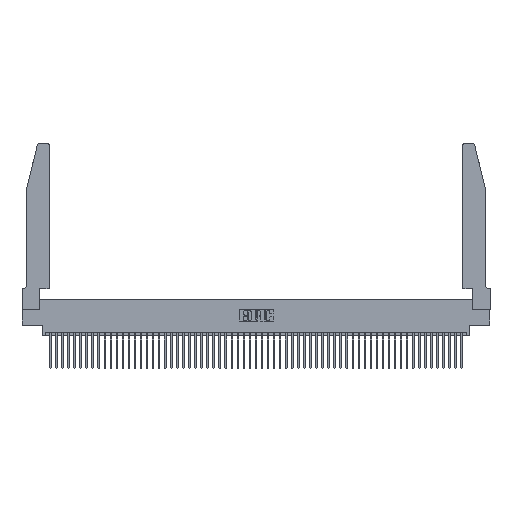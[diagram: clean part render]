
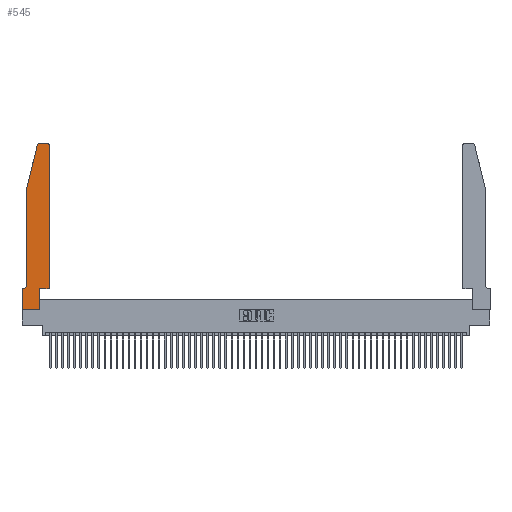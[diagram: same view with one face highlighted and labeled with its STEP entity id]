
A CAD part, top view. The second image highlights one B-rep face of the part: STEP entity #545.
In plain terms, the highlighted planar face has unit normal (0, 0, 1).
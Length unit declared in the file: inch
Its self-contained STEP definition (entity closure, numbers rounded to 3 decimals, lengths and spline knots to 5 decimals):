
#364 = CARTESIAN_POINT ( 'NONE',  ( 0.2865, 0., 0.37 ) ) ;
#421 = VERTEX_POINT ( 'NONE', #25984 ) ;
#545 = ADVANCED_FACE ( 'NONE', ( #20314 ), #48252, .T. ) ;
#788 = CARTESIAN_POINT ( 'NONE',  ( 0.4505, 0.35, 0.37 ) ) ;
#1491 = ORIENTED_EDGE ( 'NONE', *, *, #18089, .T. ) ;
#1520 = EDGE_CURVE ( 'NONE', #30617, #48166, #13519, .T. ) ;
#1555 = CARTESIAN_POINT ( 'NONE',  ( 0.2865, 0.35, 0.37 ) ) ;
#1757 = AXIS2_PLACEMENT_3D ( 'NONE', #18480, #22766, #52526 ) ;
#2494 = CARTESIAN_POINT ( 'NONE',  ( 0., 0., 0.37 ) ) ;
#3721 = LINE ( 'NONE', #34430, #25256 ) ;
#3738 = VERTEX_POINT ( 'NONE', #1555 ) ;
#3879 = CARTESIAN_POINT ( 'NONE',  ( 0.4205, 2.75, 0.37 ) ) ;
#4002 = ORIENTED_EDGE ( 'NONE', *, *, #31772, .T. ) ;
#4482 = ORIENTED_EDGE ( 'NONE', *, *, #18415, .T. ) ;
#5188 = DIRECTION ( 'NONE',  ( 1., 0., 0. ) ) ;
#5267 = LINE ( 'NONE', #51120, #28077 ) ;
#5495 = EDGE_CURVE ( 'NONE', #5815, #22100, #45076, .T. ) ;
#5815 = VERTEX_POINT ( 'NONE', #2494 ) ;
#7204 = EDGE_CURVE ( 'NONE', #14123, #5815, #22339, .T. ) ;
#8270 = DIRECTION ( 'NONE',  ( 0., 0., -1. ) ) ;
#9297 = EDGE_LOOP ( 'NONE', ( #52749, #41530, #14482, #4002, #37548, #14957, #15525, #34235, #4482, #1491, #36818, #38506 ) ) ;
#9496 = CARTESIAN_POINT ( 'NONE',  ( 0.284, 2.72, 0.37 ) ) ;
#10031 = LINE ( 'NONE', #15832, #32781 ) ;
#10834 = CARTESIAN_POINT ( 'NONE',  ( 0.0755, 2., 0.37 ) ) ;
#10952 = VECTOR ( 'NONE', #50764, 39.37008 ) ;
#11741 = LINE ( 'NONE', #48733, #54391 ) ;
#12456 = CARTESIAN_POINT ( 'NONE',  ( 0.284, 2.75, 0.37 ) ) ;
#12758 = DIRECTION ( 'NONE',  ( 0., -1., 0. ) ) ;
#13519 = CIRCLE ( 'NONE', #51260, 0.07 ) ;
#13833 = DIRECTION ( 'NONE',  ( 1., 0., 0. ) ) ;
#14123 = VERTEX_POINT ( 'NONE', #41186 ) ;
#14482 = ORIENTED_EDGE ( 'NONE', *, *, #49240, .T. ) ;
#14957 = ORIENTED_EDGE ( 'NONE', *, *, #47064, .T. ) ;
#15132 = VECTOR ( 'NONE', #38195, 39.37008 ) ;
#15156 = DIRECTION ( 'NONE',  ( -0.239, -0.971, 0. ) ) ;
#15525 = ORIENTED_EDGE ( 'NONE', *, *, #7204, .T. ) ;
#15832 = CARTESIAN_POINT ( 'NONE',  ( 0.4505, 0.35, 0.37 ) ) ;
#16935 = CARTESIAN_POINT ( 'NONE',  ( 0.4505, 0.35, 0.37 ) ) ;
#17015 = DIRECTION ( 'NONE',  ( -1., 0., 0. ) ) ;
#18089 = EDGE_CURVE ( 'NONE', #3738, #33322, #49113, .T. ) ;
#18415 = EDGE_CURVE ( 'NONE', #22100, #3738, #11741, .T. ) ;
#18480 = CARTESIAN_POINT ( 'NONE',  ( 0., 0.35, 0.37 ) ) ;
#18941 = DIRECTION ( 'NONE',  ( 0., 1., 0. ) ) ;
#20114 = DIRECTION ( 'NONE',  ( 0., 1., 0. ) ) ;
#20314 = FACE_OUTER_BOUND ( 'NONE', #9297, .T. ) ;
#21080 = CARTESIAN_POINT ( 'NONE',  ( 0.0755, 0.42, 0.37 ) ) ;
#21523 = DIRECTION ( 'NONE',  ( -1., 0., 0. ) ) ;
#21556 = VERTEX_POINT ( 'NONE', #48401 ) ;
#21779 = EDGE_CURVE ( 'NONE', #22602, #39318, #38906, .T. ) ;
#22100 = VERTEX_POINT ( 'NONE', #364 ) ;
#22298 = CARTESIAN_POINT ( 'NONE',  ( 0., 0., 0.37 ) ) ;
#22339 = LINE ( 'NONE', #33730, #10952 ) ;
#22602 = VERTEX_POINT ( 'NONE', #32327 ) ;
#22766 = DIRECTION ( 'NONE',  ( 0., 0., 1. ) ) ;
#22988 = AXIS2_PLACEMENT_3D ( 'NONE', #24372, #54117, #28657 ) ;
#23686 = LINE ( 'NONE', #29881, #45009 ) ;
#24205 = AXIS2_PLACEMENT_3D ( 'NONE', #9496, #39413, #13833 ) ;
#24372 = CARTESIAN_POINT ( 'NONE',  ( 0.4205, 2.72, 0.37 ) ) ;
#25256 = VECTOR ( 'NONE', #21523, 39.37008 ) ;
#25984 = CARTESIAN_POINT ( 'NONE',  ( 0.0755, 2., 0.37 ) ) ;
#28077 = VECTOR ( 'NONE', #12758, 39.37008 ) ;
#28409 = VECTOR ( 'NONE', #15156, 39.37008 ) ;
#28657 = DIRECTION ( 'NONE',  ( 1., 0., 0. ) ) ;
#29881 = CARTESIAN_POINT ( 'NONE',  ( 0.2605, 2.75, 0.37 ) ) ;
#30617 = VERTEX_POINT ( 'NONE', #21080 ) ;
#31772 = EDGE_CURVE ( 'NONE', #421, #30617, #5267, .T. ) ;
#32327 = CARTESIAN_POINT ( 'NONE',  ( 0.4505, 2.72, 0.37 ) ) ;
#32781 = VECTOR ( 'NONE', #20114, 39.37008 ) ;
#33322 = VERTEX_POINT ( 'NONE', #788 ) ;
#33730 = CARTESIAN_POINT ( 'NONE',  ( 0., 0., 0.37 ) ) ;
#33809 = VECTOR ( 'NONE', #5188, 39.37008 ) ;
#33929 = CARTESIAN_POINT ( 'NONE',  ( 0.0055, 0.42, 0.37 ) ) ;
#34235 = ORIENTED_EDGE ( 'NONE', *, *, #5495, .T. ) ;
#34430 = CARTESIAN_POINT ( 'NONE',  ( 0.0755, 0.35, 0.37 ) ) ;
#36818 = ORIENTED_EDGE ( 'NONE', *, *, #45265, .T. ) ;
#37548 = ORIENTED_EDGE ( 'NONE', *, *, #1520, .T. ) ;
#38195 = DIRECTION ( 'NONE',  ( 1., 0., 0. ) ) ;
#38199 = DIRECTION ( 'NONE',  ( -1., 0., 0. ) ) ;
#38506 = ORIENTED_EDGE ( 'NONE', *, *, #21779, .T. ) ;
#38906 = CIRCLE ( 'NONE', #22988, 0.03 ) ;
#39318 = VERTEX_POINT ( 'NONE', #3879 ) ;
#39413 = DIRECTION ( 'NONE',  ( 0., 0., 1. ) ) ;
#39986 = EDGE_CURVE ( 'NONE', #42653, #21556, #40830, .T. ) ;
#40830 = CIRCLE ( 'NONE', #24205, 0.03 ) ;
#41186 = CARTESIAN_POINT ( 'NONE',  ( 0., 0.35, 0.37 ) ) ;
#41530 = ORIENTED_EDGE ( 'NONE', *, *, #39986, .T. ) ;
#42653 = VERTEX_POINT ( 'NONE', #12456 ) ;
#45009 = VECTOR ( 'NONE', #17015, 39.37008 ) ;
#45076 = LINE ( 'NONE', #22298, #33809 ) ;
#45265 = EDGE_CURVE ( 'NONE', #33322, #22602, #10031, .T. ) ;
#45792 = CARTESIAN_POINT ( 'NONE',  ( 0.0055, 0.35, 0.37 ) ) ;
#47064 = EDGE_CURVE ( 'NONE', #48166, #14123, #3721, .T. ) ;
#48166 = VERTEX_POINT ( 'NONE', #45792 ) ;
#48252 = PLANE ( 'NONE',  #1757 ) ;
#48401 = CARTESIAN_POINT ( 'NONE',  ( 0.25487, 2.72718, 0.37 ) ) ;
#48733 = CARTESIAN_POINT ( 'NONE',  ( 0.2865, 0.35, 0.37 ) ) ;
#49113 = LINE ( 'NONE', #16935, #15132 ) ;
#49240 = EDGE_CURVE ( 'NONE', #21556, #421, #50251, .T. ) ;
#49559 = EDGE_CURVE ( 'NONE', #39318, #42653, #23686, .T. ) ;
#50251 = LINE ( 'NONE', #10834, #28409 ) ;
#50764 = DIRECTION ( 'NONE',  ( 0., -1., 0. ) ) ;
#51120 = CARTESIAN_POINT ( 'NONE',  ( 0.0755, 2., 0.37 ) ) ;
#51260 = AXIS2_PLACEMENT_3D ( 'NONE', #33929, #8270, #38199 ) ;
#52526 = DIRECTION ( 'NONE',  ( 1., 0., 0. ) ) ;
#52749 = ORIENTED_EDGE ( 'NONE', *, *, #49559, .T. ) ;
#54117 = DIRECTION ( 'NONE',  ( 0., 0., 1. ) ) ;
#54391 = VECTOR ( 'NONE', #18941, 39.37008 ) ;
